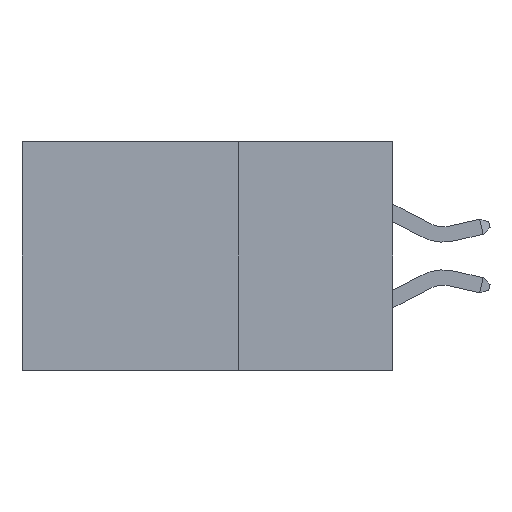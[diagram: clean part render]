
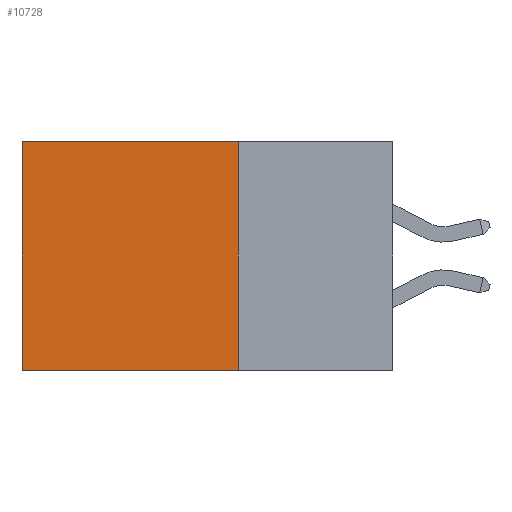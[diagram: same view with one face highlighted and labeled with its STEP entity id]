
A CAD part, left-side view. The second image highlights one B-rep face of the part: STEP entity #10728.
In plain terms, the highlighted planar face has unit normal (-1, 0, 0).
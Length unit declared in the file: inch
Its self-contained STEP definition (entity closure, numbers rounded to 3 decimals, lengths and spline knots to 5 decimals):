
#1644 = DIRECTION ( 'NONE',  ( 0., 0., -1. ) ) ;
#1689 = VECTOR ( 'NONE', #13358, 39.37008 ) ;
#2187 = FACE_OUTER_BOUND ( 'NONE', #36895, .T. ) ;
#2755 = CARTESIAN_POINT ( 'NONE',  ( 0.2875, 0.25, -0.37 ) ) ;
#3035 = EDGE_CURVE ( 'NONE', #16400, #28218, #21797, .T. ) ;
#3858 = VECTOR ( 'NONE', #10816, 39.37008 ) ;
#4344 = CARTESIAN_POINT ( 'NONE',  ( 0.2875, 0.6, 0. ) ) ;
#5370 = LINE ( 'NONE', #14460, #6368 ) ;
#6123 = AXIS2_PLACEMENT_3D ( 'NONE', #39420, #20792, #1644 ) ;
#6368 = VECTOR ( 'NONE', #33177, 39.37008 ) ;
#9336 = EDGE_CURVE ( 'NONE', #39290, #32865, #5370, .T. ) ;
#10728 = ADVANCED_FACE ( 'NONE', ( #2187 ), #33144, .F. ) ;
#10816 = DIRECTION ( 'NONE',  ( 0., 0., -1. ) ) ;
#11876 = CARTESIAN_POINT ( 'NONE',  ( 0.2875, 0.6, 0. ) ) ;
#13358 = DIRECTION ( 'NONE',  ( 0., 1., 0. ) ) ;
#14460 = CARTESIAN_POINT ( 'NONE',  ( 0.2875, 0.25, 0. ) ) ;
#16400 = VERTEX_POINT ( 'NONE', #11876 ) ;
#18579 = CARTESIAN_POINT ( 'NONE',  ( 0.2875, 0.25, -0.37 ) ) ;
#18759 = LINE ( 'NONE', #22722, #1689 ) ;
#18888 = VECTOR ( 'NONE', #31079, 39.37008 ) ;
#18982 = EDGE_CURVE ( 'NONE', #39290, #16400, #18759, .T. ) ;
#20497 = ORIENTED_EDGE ( 'NONE', *, *, #3035, .T. ) ;
#20792 = DIRECTION ( 'NONE',  ( 1., 0., 0. ) ) ;
#21797 = LINE ( 'NONE', #4344, #3858 ) ;
#22722 = CARTESIAN_POINT ( 'NONE',  ( 0.2875, 0.25, 0. ) ) ;
#23748 = CARTESIAN_POINT ( 'NONE',  ( 0.2875, 0.25, 0. ) ) ;
#23892 = ORIENTED_EDGE ( 'NONE', *, *, #30082, .F. ) ;
#28218 = VERTEX_POINT ( 'NONE', #37903 ) ;
#30082 = EDGE_CURVE ( 'NONE', #32865, #28218, #34455, .T. ) ;
#31079 = DIRECTION ( 'NONE',  ( 0., 1., 0. ) ) ;
#31283 = ORIENTED_EDGE ( 'NONE', *, *, #9336, .F. ) ;
#32865 = VERTEX_POINT ( 'NONE', #2755 ) ;
#33144 = PLANE ( 'NONE',  #6123 ) ;
#33177 = DIRECTION ( 'NONE',  ( 0., 0., -1. ) ) ;
#34455 = LINE ( 'NONE', #18579, #18888 ) ;
#36895 = EDGE_LOOP ( 'NONE', ( #20497, #23892, #31283, #38076 ) ) ;
#37903 = CARTESIAN_POINT ( 'NONE',  ( 0.2875, 0.6, -0.37 ) ) ;
#38076 = ORIENTED_EDGE ( 'NONE', *, *, #18982, .T. ) ;
#39290 = VERTEX_POINT ( 'NONE', #23748 ) ;
#39420 = CARTESIAN_POINT ( 'NONE',  ( 0.2875, 0.25, 0. ) ) ;
